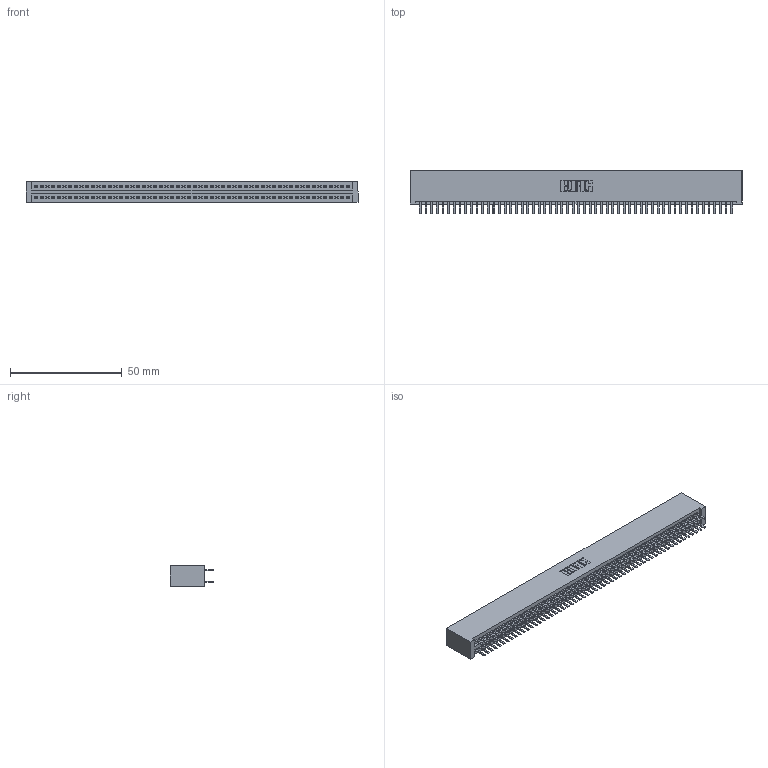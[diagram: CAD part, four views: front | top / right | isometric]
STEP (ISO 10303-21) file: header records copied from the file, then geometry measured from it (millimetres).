
FILE_DESCRIPTION (( 'STEP AP203' ), '1' );
FILE_NAME ('345-112-520-201.STEP', '2018-10-07T13:26:17', ( '' ), ( '' ), 'SwSTEP 2.0', 'SolidWorks 2016', '' );
FILE_SCHEMA (( 'CONFIG_CONTROL_DESIGN' ));
Length unit declared in the file: inch
Products named in the file (3): 345-292-001_345-293-120; 345-112-520-201; 345 Part_No Mounting Lugs
Assembly tree (113 placements, depth 2):
  345-112-520-201
    345 Part_No Mounting Lugs
    345-292-001_345-293-120  x112
Bounding box: 148.84 x 19.68 x 9.4 mm (x, y, z)
Volume: 15155.5 mm3; surface area: 22872 mm2
Topology: 113 solids, 113 shells, 6166 faces, 17901 edges, 11634 vertices
Faces by surface type: plane 3996, cylinder 2170
Entity records: 41891 total; most frequent: CARTESIAN_POINT 7020, ORIENTED_EDGE 6942, DIRECTION 6155, EDGE_CURVE 3471, LINE 3119, VECTOR 3119, VERTEX_POINT 2310, AXIS2_PLACEMENT_3D 1518
